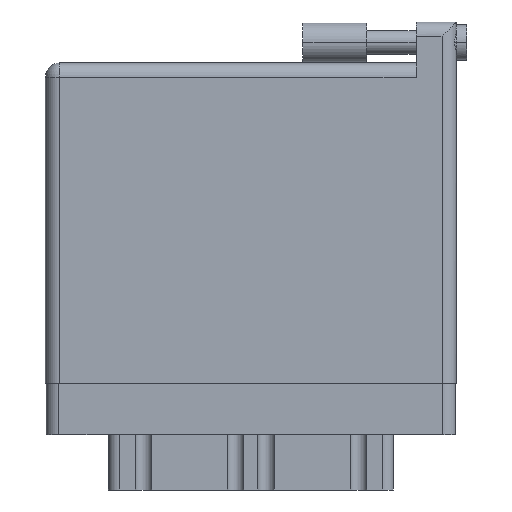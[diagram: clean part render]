
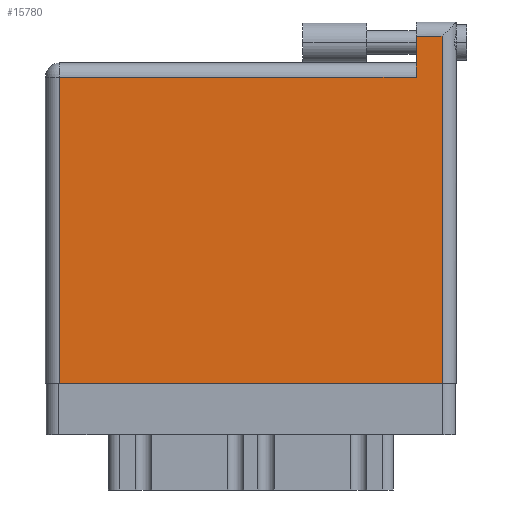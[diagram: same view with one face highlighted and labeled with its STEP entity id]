
A CAD part, front view. The second image highlights one B-rep face of the part: STEP entity #15780.
In plain terms, the highlighted face is planar.
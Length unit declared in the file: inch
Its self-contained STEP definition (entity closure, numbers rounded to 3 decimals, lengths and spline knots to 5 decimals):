
#1084 = EDGE_CURVE ( 'NONE', #3481, #16668, #29838, .T. ) ;
#1172 = AXIS2_PLACEMENT_3D ( 'NONE', #26043, #14198, #37926 ) ;
#2624 = VECTOR ( 'NONE', #18335, 39.37008 ) ;
#2768 = DIRECTION ( 'NONE',  ( -1., 0., 0. ) ) ;
#2851 = CARTESIAN_POINT ( 'NONE',  ( 1.938, 1.766, 0. ) ) ;
#3178 = VECTOR ( 'NONE', #2768, 39.37008 ) ;
#3481 = VERTEX_POINT ( 'NONE', #32635 ) ;
#4176 = CARTESIAN_POINT ( 'NONE',  ( 0.07, 0., 0. ) ) ;
#5734 = LINE ( 'NONE', #15111, #9926 ) ;
#5926 = VERTEX_POINT ( 'NONE', #28974 ) ;
#6954 = ORIENTED_EDGE ( 'NONE', *, *, #32061, .T. ) ;
#7185 = VERTEX_POINT ( 'NONE', #33121 ) ;
#8689 = VECTOR ( 'NONE', #18233, 39.37008 ) ;
#8889 = LINE ( 'NONE', #2851, #8689 ) ;
#9926 = VECTOR ( 'NONE', #14540, 39.37008 ) ;
#10024 = ORIENTED_EDGE ( 'NONE', *, *, #31610, .T. ) ;
#10338 = EDGE_CURVE ( 'NONE', #7185, #18846, #28638, .T. ) ;
#12874 = VECTOR ( 'NONE', #20912, 39.37008 ) ;
#14198 = DIRECTION ( 'NONE',  ( 0., 0., -1. ) ) ;
#14540 = DIRECTION ( 'NONE',  ( -1., 0., 0. ) ) ;
#14910 = ORIENTED_EDGE ( 'NONE', *, *, #19899, .T. ) ;
#14927 = ORIENTED_EDGE ( 'NONE', *, *, #36674, .T. ) ;
#15111 = CARTESIAN_POINT ( 'NONE',  ( 0., 1.696, 0. ) ) ;
#15780 = ADVANCED_FACE ( 'NONE', ( #20599 ), #29545, .F. ) ;
#16668 = VERTEX_POINT ( 'NONE', #27237 ) ;
#16982 = EDGE_LOOP ( 'NONE', ( #14927, #6954, #10024, #22274, #14910, #24291 ) ) ;
#18233 = DIRECTION ( 'NONE',  ( 0., 1., 0. ) ) ;
#18335 = DIRECTION ( 'NONE',  ( 1., 0., 0. ) ) ;
#18846 = VERTEX_POINT ( 'NONE', #4176 ) ;
#19899 = EDGE_CURVE ( 'NONE', #16668, #7185, #29053, .T. ) ;
#20599 = FACE_OUTER_BOUND ( 'NONE', #16982, .T. ) ;
#20912 = DIRECTION ( 'NONE',  ( 0., -1., 0. ) ) ;
#21247 = LINE ( 'NONE', #33101, #2624 ) ;
#22274 = ORIENTED_EDGE ( 'NONE', *, *, #1084, .T. ) ;
#22793 = CARTESIAN_POINT ( 'NONE',  ( 1.938, 1.696, 0. ) ) ;
#24291 = ORIENTED_EDGE ( 'NONE', *, *, #10338, .T. ) ;
#26043 = CARTESIAN_POINT ( 'NONE',  ( 0., 1.566, 0. ) ) ;
#27237 = CARTESIAN_POINT ( 'NONE',  ( 1.811, 1.496, 0. ) ) ;
#28638 = LINE ( 'NONE', #37404, #33567 ) ;
#28974 = CARTESIAN_POINT ( 'NONE',  ( 1.938, 0., 0. ) ) ;
#29053 = LINE ( 'NONE', #29440, #3178 ) ;
#29440 = CARTESIAN_POINT ( 'NONE',  ( 0., 1.496, 0. ) ) ;
#29545 = PLANE ( 'NONE',  #1172 ) ;
#29838 = LINE ( 'NONE', #33149, #12874 ) ;
#31610 = EDGE_CURVE ( 'NONE', #38039, #3481, #5734, .T. ) ;
#32061 = EDGE_CURVE ( 'NONE', #5926, #38039, #8889, .T. ) ;
#32635 = CARTESIAN_POINT ( 'NONE',  ( 1.811, 1.696, 0. ) ) ;
#33101 = CARTESIAN_POINT ( 'NONE',  ( 0., 0., 0. ) ) ;
#33121 = CARTESIAN_POINT ( 'NONE',  ( 0.07, 1.496, 0. ) ) ;
#33149 = CARTESIAN_POINT ( 'NONE',  ( 1.811, 1.766, 0. ) ) ;
#33567 = VECTOR ( 'NONE', #34667, 39.37008 ) ;
#34667 = DIRECTION ( 'NONE',  ( 0., -1., 0. ) ) ;
#36674 = EDGE_CURVE ( 'NONE', #18846, #5926, #21247, .T. ) ;
#37404 = CARTESIAN_POINT ( 'NONE',  ( 0.07, 0., 0. ) ) ;
#37926 = DIRECTION ( 'NONE',  ( -1., 0., 0. ) ) ;
#38039 = VERTEX_POINT ( 'NONE', #22793 ) ;
